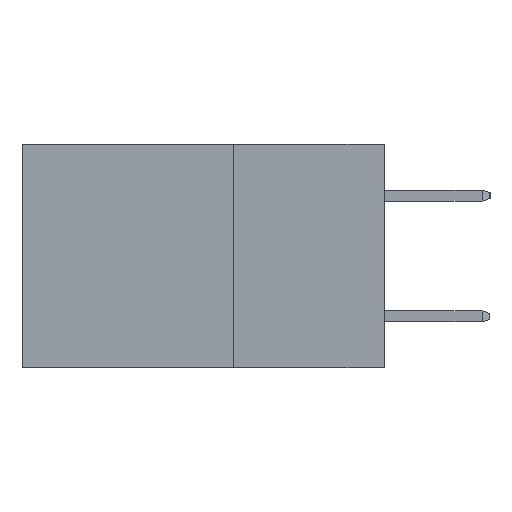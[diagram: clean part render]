
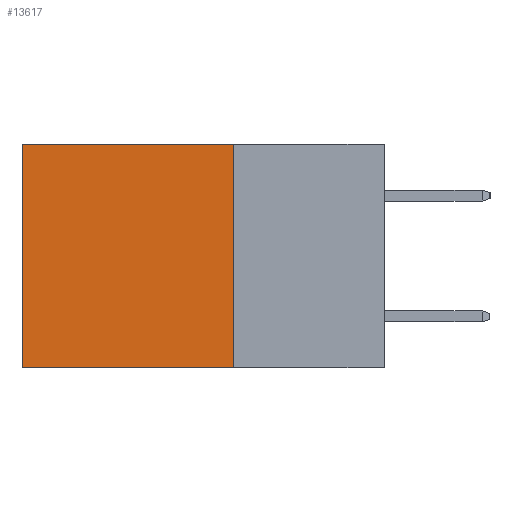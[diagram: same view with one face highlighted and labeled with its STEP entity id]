
A CAD part, left-side view. The second image highlights one B-rep face of the part: STEP entity #13617.
In plain terms, the highlighted planar face has unit normal (-1, 0, 0).
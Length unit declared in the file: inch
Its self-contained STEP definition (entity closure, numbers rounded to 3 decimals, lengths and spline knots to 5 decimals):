
#278 = DIRECTION ( 'NONE',  ( 0., 1., 0. ) ) ;
#1803 = CARTESIAN_POINT ( 'NONE',  ( 0.298, 0.6, -0.37 ) ) ;
#2049 = ORIENTED_EDGE ( 'NONE', *, *, #4103, .T. ) ;
#3350 = EDGE_CURVE ( 'NONE', #13157, #9190, #5378, .T. ) ;
#3988 = ORIENTED_EDGE ( 'NONE', *, *, #5910, .T. ) ;
#4103 = EDGE_CURVE ( 'NONE', #9288, #5968, #10633, .T. ) ;
#4867 = VECTOR ( 'NONE', #16887, 39.37008 ) ;
#5133 = CARTESIAN_POINT ( 'NONE',  ( 0.298, 0.25, -0.37 ) ) ;
#5306 = CARTESIAN_POINT ( 'NONE',  ( 0.298, 0.6, 0. ) ) ;
#5378 = LINE ( 'NONE', #8498, #12318 ) ;
#5382 = DIRECTION ( 'NONE',  ( 0., 0., -1. ) ) ;
#5777 = CARTESIAN_POINT ( 'NONE',  ( 0.298, 0.25, 0. ) ) ;
#5910 = EDGE_CURVE ( 'NONE', #13157, #9288, #11646, .T. ) ;
#5968 = VERTEX_POINT ( 'NONE', #1803 ) ;
#7118 = ORIENTED_EDGE ( 'NONE', *, *, #7482, .F. ) ;
#7221 = ORIENTED_EDGE ( 'NONE', *, *, #3350, .F. ) ;
#7482 = EDGE_CURVE ( 'NONE', #9190, #5968, #15433, .T. ) ;
#8031 = VECTOR ( 'NONE', #278, 39.37008 ) ;
#8204 = CARTESIAN_POINT ( 'NONE',  ( 0.298, 0.25, 0. ) ) ;
#8498 = CARTESIAN_POINT ( 'NONE',  ( 0.298, 0.25, 0. ) ) ;
#9190 = VERTEX_POINT ( 'NONE', #5133 ) ;
#9288 = VERTEX_POINT ( 'NONE', #5306 ) ;
#10168 = EDGE_LOOP ( 'NONE', ( #2049, #7118, #7221, #3988 ) ) ;
#10274 = FACE_OUTER_BOUND ( 'NONE', #10168, .T. ) ;
#10633 = LINE ( 'NONE', #12093, #17005 ) ;
#10859 = AXIS2_PLACEMENT_3D ( 'NONE', #8204, #13646, #5382 ) ;
#11294 = CARTESIAN_POINT ( 'NONE',  ( 0.298, 0.25, 0. ) ) ;
#11646 = LINE ( 'NONE', #5777, #8031 ) ;
#12093 = CARTESIAN_POINT ( 'NONE',  ( 0.298, 0.6, 0. ) ) ;
#12318 = VECTOR ( 'NONE', #15588, 39.37008 ) ;
#12837 = DIRECTION ( 'NONE',  ( 0., 0., -1. ) ) ;
#13157 = VERTEX_POINT ( 'NONE', #11294 ) ;
#13617 = ADVANCED_FACE ( 'NONE', ( #10274 ), #17690, .F. ) ;
#13646 = DIRECTION ( 'NONE',  ( 1., 0., 0. ) ) ;
#14182 = CARTESIAN_POINT ( 'NONE',  ( 0.298, 0.25, -0.37 ) ) ;
#15433 = LINE ( 'NONE', #14182, #4867 ) ;
#15588 = DIRECTION ( 'NONE',  ( 0., 0., -1. ) ) ;
#16887 = DIRECTION ( 'NONE',  ( 0., 1., 0. ) ) ;
#17005 = VECTOR ( 'NONE', #12837, 39.37008 ) ;
#17690 = PLANE ( 'NONE',  #10859 ) ;
